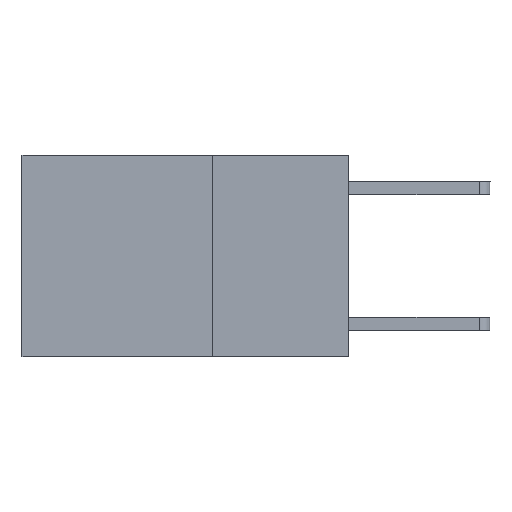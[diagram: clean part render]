
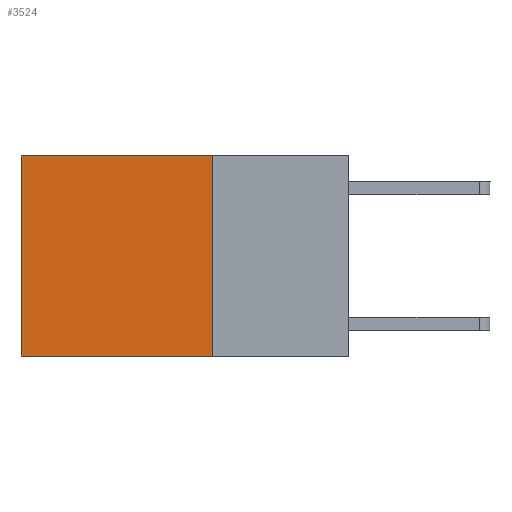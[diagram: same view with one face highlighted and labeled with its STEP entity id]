
A CAD part, left-side view. The second image highlights one B-rep face of the part: STEP entity #3524.
In plain terms, the highlighted planar face has unit normal (-1, 0, 0).
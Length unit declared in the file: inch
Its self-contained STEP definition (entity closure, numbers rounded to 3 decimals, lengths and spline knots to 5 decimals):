
#27 = CARTESIAN_POINT ( 'NONE',  ( 0.2625, 0.25, 0. ) ) ;
#76 = VERTEX_POINT ( 'NONE', #8733 ) ;
#601 = DIRECTION ( 'NONE',  ( 0., 0., -1. ) ) ;
#860 = ORIENTED_EDGE ( 'NONE', *, *, #6101, .T. ) ;
#1362 = LINE ( 'NONE', #4295, #6419 ) ;
#2663 = CARTESIAN_POINT ( 'NONE',  ( 0.2625, 0.6, 0. ) ) ;
#2823 = EDGE_LOOP ( 'NONE', ( #3890, #6852, #5537, #860 ) ) ;
#3028 = CARTESIAN_POINT ( 'NONE',  ( 0.2625, 0.6, 0. ) ) ;
#3524 = ADVANCED_FACE ( 'NONE', ( #4404 ), #7342, .F. ) ;
#3700 = VERTEX_POINT ( 'NONE', #2663 ) ;
#3890 = ORIENTED_EDGE ( 'NONE', *, *, #6143, .T. ) ;
#4043 = VERTEX_POINT ( 'NONE', #4785 ) ;
#4094 = VECTOR ( 'NONE', #6954, 39.37008 ) ;
#4219 = CARTESIAN_POINT ( 'NONE',  ( 0.2625, 0.25, 0. ) ) ;
#4295 = CARTESIAN_POINT ( 'NONE',  ( 0.2625, 0.25, 0. ) ) ;
#4395 = LINE ( 'NONE', #27, #4585 ) ;
#4404 = FACE_OUTER_BOUND ( 'NONE', #2823, .T. ) ;
#4440 = LINE ( 'NONE', #3028, #6719 ) ;
#4585 = VECTOR ( 'NONE', #6646, 39.37008 ) ;
#4776 = CARTESIAN_POINT ( 'NONE',  ( 0.2625, 0.25, -0.37 ) ) ;
#4785 = CARTESIAN_POINT ( 'NONE',  ( 0.2625, 0.6, -0.37 ) ) ;
#4827 = AXIS2_PLACEMENT_3D ( 'NONE', #4219, #7129, #601 ) ;
#4878 = LINE ( 'NONE', #4776, #4094 ) ;
#5537 = ORIENTED_EDGE ( 'NONE', *, *, #6594, .F. ) ;
#6101 = EDGE_CURVE ( 'NONE', #7836, #3700, #1362, .T. ) ;
#6143 = EDGE_CURVE ( 'NONE', #3700, #4043, #4440, .T. ) ;
#6419 = VECTOR ( 'NONE', #7226, 39.37008 ) ;
#6594 = EDGE_CURVE ( 'NONE', #7836, #76, #4395, .T. ) ;
#6646 = DIRECTION ( 'NONE',  ( 0., 0., -1. ) ) ;
#6719 = VECTOR ( 'NONE', #7413, 39.37008 ) ;
#6852 = ORIENTED_EDGE ( 'NONE', *, *, #8035, .F. ) ;
#6954 = DIRECTION ( 'NONE',  ( 0., 1., 0. ) ) ;
#7129 = DIRECTION ( 'NONE',  ( 1., 0., 0. ) ) ;
#7226 = DIRECTION ( 'NONE',  ( 0., 1., 0. ) ) ;
#7342 = PLANE ( 'NONE',  #4827 ) ;
#7413 = DIRECTION ( 'NONE',  ( 0., 0., -1. ) ) ;
#7836 = VERTEX_POINT ( 'NONE', #8380 ) ;
#8035 = EDGE_CURVE ( 'NONE', #76, #4043, #4878, .T. ) ;
#8380 = CARTESIAN_POINT ( 'NONE',  ( 0.2625, 0.25, 0. ) ) ;
#8733 = CARTESIAN_POINT ( 'NONE',  ( 0.2625, 0.25, -0.37 ) ) ;
